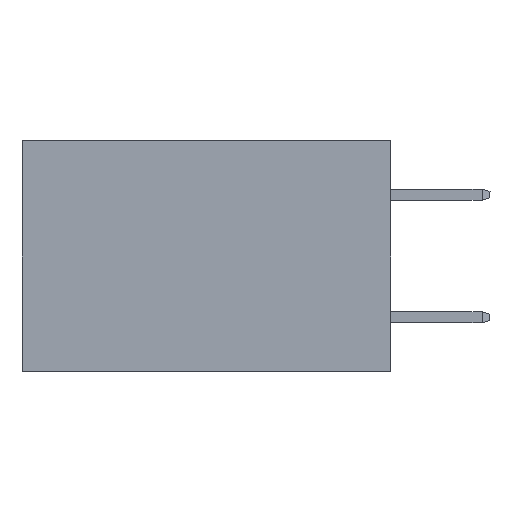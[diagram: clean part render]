
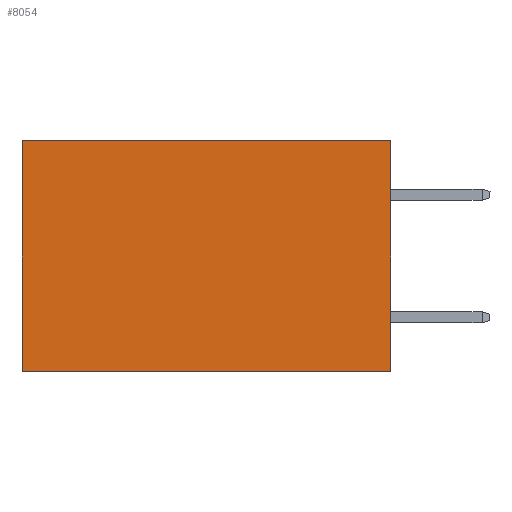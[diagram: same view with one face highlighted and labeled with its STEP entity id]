
A CAD part, left-side view. The second image highlights one B-rep face of the part: STEP entity #8054.
In plain terms, the highlighted planar face has unit normal (-1, 0, 0).
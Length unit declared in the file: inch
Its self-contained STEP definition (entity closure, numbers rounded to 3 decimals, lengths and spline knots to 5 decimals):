
#114 = VERTEX_POINT ( 'NONE', #7845 ) ;
#314 = CARTESIAN_POINT ( 'NONE',  ( 0.2875, 0.6, -0.375 ) ) ;
#342 = DIRECTION ( 'NONE',  ( 0., 0., -1. ) ) ;
#438 = CARTESIAN_POINT ( 'NONE',  ( 0.2875, 0., -0.375 ) ) ;
#522 = DIRECTION ( 'NONE',  ( 0., 0., -1. ) ) ;
#1162 = PLANE ( 'NONE',  #4556 ) ;
#1291 = CARTESIAN_POINT ( 'NONE',  ( 0.2875, 0., 0. ) ) ;
#1423 = VECTOR ( 'NONE', #342, 39.37008 ) ;
#1524 = VECTOR ( 'NONE', #6409, 39.37008 ) ;
#2019 = VERTEX_POINT ( 'NONE', #2647 ) ;
#2288 = LINE ( 'NONE', #6435, #5159 ) ;
#2498 = VECTOR ( 'NONE', #6866, 39.37008 ) ;
#2513 = VERTEX_POINT ( 'NONE', #7746 ) ;
#2533 = EDGE_CURVE ( 'NONE', #2513, #2019, #2288, .T. ) ;
#2568 = EDGE_LOOP ( 'NONE', ( #7465, #5004, #3886, #7735 ) ) ;
#2647 = CARTESIAN_POINT ( 'NONE',  ( 0.2875, 0., -0.375 ) ) ;
#3112 = DIRECTION ( 'NONE',  ( 1., 0., 0. ) ) ;
#3302 = DIRECTION ( 'NONE',  ( 0., 0., -1. ) ) ;
#3331 = LINE ( 'NONE', #314, #1423 ) ;
#3805 = LINE ( 'NONE', #4210, #2498 ) ;
#3886 = ORIENTED_EDGE ( 'NONE', *, *, #2533, .F. ) ;
#4177 = VERTEX_POINT ( 'NONE', #4367 ) ;
#4210 = CARTESIAN_POINT ( 'NONE',  ( 0.2875, 0., -0.375 ) ) ;
#4367 = CARTESIAN_POINT ( 'NONE',  ( 0.2875, 0.6, -0.375 ) ) ;
#4459 = EDGE_CURVE ( 'NONE', #114, #4177, #3331, .T. ) ;
#4556 = AXIS2_PLACEMENT_3D ( 'NONE', #438, #3112, #522 ) ;
#4691 = EDGE_CURVE ( 'NONE', #2513, #114, #5817, .T. ) ;
#5004 = ORIENTED_EDGE ( 'NONE', *, *, #6276, .F. ) ;
#5159 = VECTOR ( 'NONE', #3302, 39.37008 ) ;
#5817 = LINE ( 'NONE', #1291, #1524 ) ;
#6276 = EDGE_CURVE ( 'NONE', #2019, #4177, #3805, .T. ) ;
#6409 = DIRECTION ( 'NONE',  ( 0., 1., 0. ) ) ;
#6435 = CARTESIAN_POINT ( 'NONE',  ( 0.2875, 0., -0.375 ) ) ;
#6866 = DIRECTION ( 'NONE',  ( 0., 1., 0. ) ) ;
#7465 = ORIENTED_EDGE ( 'NONE', *, *, #4459, .T. ) ;
#7591 = FACE_OUTER_BOUND ( 'NONE', #2568, .T. ) ;
#7735 = ORIENTED_EDGE ( 'NONE', *, *, #4691, .T. ) ;
#7746 = CARTESIAN_POINT ( 'NONE',  ( 0.2875, 0., 0. ) ) ;
#7845 = CARTESIAN_POINT ( 'NONE',  ( 0.2875, 0.6, 0. ) ) ;
#8054 = ADVANCED_FACE ( 'NONE', ( #7591 ), #1162, .F. ) ;
